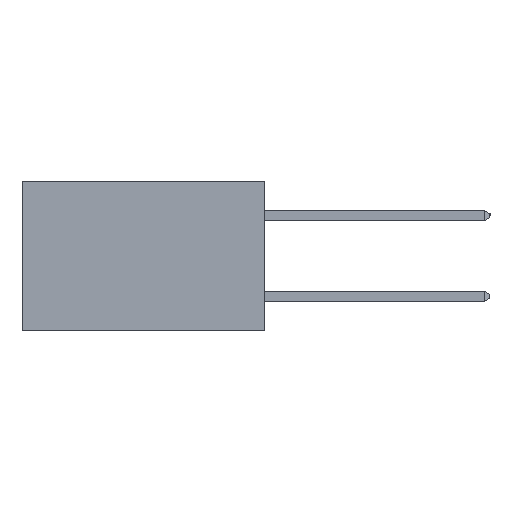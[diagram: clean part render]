
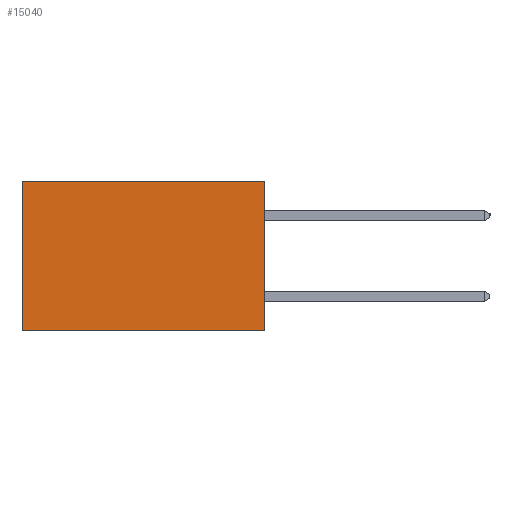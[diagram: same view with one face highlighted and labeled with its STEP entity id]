
A CAD part, left-side view. The second image highlights one B-rep face of the part: STEP entity #15040.
In plain terms, the highlighted planar face has unit normal (-1, 0, 0).
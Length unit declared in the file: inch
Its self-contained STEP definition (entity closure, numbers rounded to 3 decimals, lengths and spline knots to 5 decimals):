
#237 = DIRECTION ( 'NONE',  ( 1., 0., 0. ) ) ;
#260 = EDGE_CURVE ( 'NONE', #21022, #14192, #4562, .T. ) ;
#526 = VERTEX_POINT ( 'NONE', #8316 ) ;
#782 = EDGE_CURVE ( 'NONE', #526, #14192, #8177, .T. ) ;
#789 = AXIS2_PLACEMENT_3D ( 'NONE', #10901, #237, #12653 ) ;
#1515 = CARTESIAN_POINT ( 'NONE',  ( 0.298, 0., -0.37 ) ) ;
#2250 = FACE_OUTER_BOUND ( 'NONE', #13317, .T. ) ;
#4426 = CARTESIAN_POINT ( 'NONE',  ( 0.298, 0.6, -0.37 ) ) ;
#4562 = LINE ( 'NONE', #12353, #13968 ) ;
#4608 = VERTEX_POINT ( 'NONE', #21189 ) ;
#4698 = VECTOR ( 'NONE', #16171, 39.37008 ) ;
#5401 = VECTOR ( 'NONE', #16800, 39.37008 ) ;
#5803 = ORIENTED_EDGE ( 'NONE', *, *, #9450, .T. ) ;
#6745 = EDGE_CURVE ( 'NONE', #4608, #21022, #14746, .T. ) ;
#8177 = LINE ( 'NONE', #8305, #16920 ) ;
#8305 = CARTESIAN_POINT ( 'NONE',  ( 0.298, 0.6, 0. ) ) ;
#8316 = CARTESIAN_POINT ( 'NONE',  ( 0.298, 0.6, 0. ) ) ;
#8330 = DIRECTION ( 'NONE',  ( 0., 0., -1. ) ) ;
#8427 = CARTESIAN_POINT ( 'NONE',  ( 0.298, 0., 0. ) ) ;
#9450 = EDGE_CURVE ( 'NONE', #4608, #526, #19759, .T. ) ;
#10901 = CARTESIAN_POINT ( 'NONE',  ( 0.298, 0., 0. ) ) ;
#11331 = DIRECTION ( 'NONE',  ( 0., 1., 0. ) ) ;
#12353 = CARTESIAN_POINT ( 'NONE',  ( 0.298, 0., -0.37 ) ) ;
#12653 = DIRECTION ( 'NONE',  ( 0., 0., -1. ) ) ;
#13317 = EDGE_LOOP ( 'NONE', ( #21150, #22072, #16652, #5803 ) ) ;
#13968 = VECTOR ( 'NONE', #11331, 39.37008 ) ;
#14192 = VERTEX_POINT ( 'NONE', #4426 ) ;
#14746 = LINE ( 'NONE', #21323, #5401 ) ;
#15040 = ADVANCED_FACE ( 'NONE', ( #2250 ), #21251, .F. ) ;
#16171 = DIRECTION ( 'NONE',  ( 0., 1., 0. ) ) ;
#16652 = ORIENTED_EDGE ( 'NONE', *, *, #6745, .F. ) ;
#16800 = DIRECTION ( 'NONE',  ( 0., 0., -1. ) ) ;
#16920 = VECTOR ( 'NONE', #8330, 39.37008 ) ;
#19759 = LINE ( 'NONE', #8427, #4698 ) ;
#21022 = VERTEX_POINT ( 'NONE', #1515 ) ;
#21150 = ORIENTED_EDGE ( 'NONE', *, *, #782, .T. ) ;
#21189 = CARTESIAN_POINT ( 'NONE',  ( 0.298, 0., 0. ) ) ;
#21251 = PLANE ( 'NONE',  #789 ) ;
#21323 = CARTESIAN_POINT ( 'NONE',  ( 0.298, 0., 0. ) ) ;
#22072 = ORIENTED_EDGE ( 'NONE', *, *, #260, .F. ) ;
